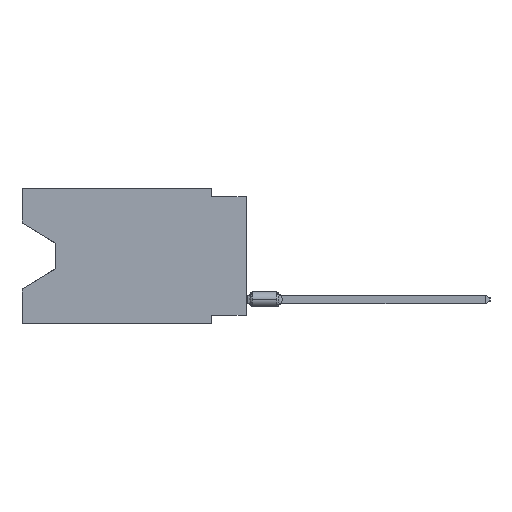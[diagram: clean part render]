
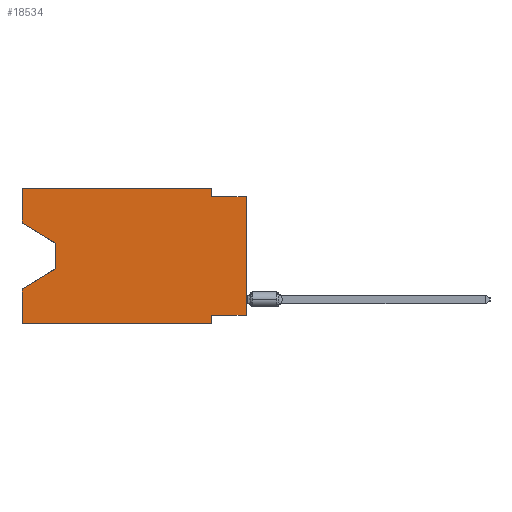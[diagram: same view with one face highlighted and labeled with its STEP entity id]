
A CAD part, left-side view. The second image highlights one B-rep face of the part: STEP entity #18534.
In plain terms, the highlighted planar face has unit normal (-1, 0, 0).
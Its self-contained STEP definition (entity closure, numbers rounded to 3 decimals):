
#212 = DIRECTION ( 'NONE',  ( 0., 0., -1. ) ) ;
#565 = EDGE_LOOP ( 'NONE', ( #54217, #32923, #70954, #8708, #57684, #69828, #55355, #9778, #17745, #63769, #45177, #51596 ) ) ;
#2578 = VECTOR ( 'NONE', #21114, 1000. ) ;
#3124 = VERTEX_POINT ( 'NONE', #63238 ) ;
#4812 = LINE ( 'NONE', #26596, #66347 ) ;
#5333 = VECTOR ( 'NONE', #43111, 1000. ) ;
#5863 = EDGE_CURVE ( 'NONE', #13954, #42335, #4812, .T. ) ;
#6368 = EDGE_CURVE ( 'NONE', #13954, #55034, #64513, .T. ) ;
#7191 = DIRECTION ( 'NONE',  ( 0., 0., 1. ) ) ;
#8708 = ORIENTED_EDGE ( 'NONE', *, *, #12662, .F. ) ;
#9778 = ORIENTED_EDGE ( 'NONE', *, *, #5863, .T. ) ;
#10524 = CARTESIAN_POINT ( 'NONE',  ( 0., 13.97, -5.893 ) ) ;
#10916 = VECTOR ( 'NONE', #31590, 1000. ) ;
#11325 = EDGE_CURVE ( 'NONE', #37197, #21861, #41984, .T. ) ;
#12066 = VECTOR ( 'NONE', #18634, 1000. ) ;
#12659 = CARTESIAN_POINT ( 'NONE',  ( 0., 16.383, -2.546 ) ) ;
#12662 = EDGE_CURVE ( 'NONE', #3124, #21861, #57821, .T. ) ;
#13291 = DIRECTION ( 'NONE',  ( 1., 0., 0. ) ) ;
#13871 = DIRECTION ( 'NONE',  ( 0., 1., 0. ) ) ;
#13954 = VERTEX_POINT ( 'NONE', #42633 ) ;
#14108 = VECTOR ( 'NONE', #62204, 1000. ) ;
#17097 = LINE ( 'NONE', #12659, #14108 ) ;
#17745 = ORIENTED_EDGE ( 'NONE', *, *, #31429, .F. ) ;
#18082 = LINE ( 'NONE', #69478, #70165 ) ;
#18534 = ADVANCED_FACE ( 'NONE', ( #29902 ), #41381, .F. ) ;
#18634 = DIRECTION ( 'NONE',  ( 0., -1., 0. ) ) ;
#18789 = LINE ( 'NONE', #30231, #33680 ) ;
#21114 = DIRECTION ( 'NONE',  ( 0., 0., 1. ) ) ;
#21443 = VERTEX_POINT ( 'NONE', #50872 ) ;
#21612 = LINE ( 'NONE', #39372, #64650 ) ;
#21861 = VERTEX_POINT ( 'NONE', #69190 ) ;
#22777 = EDGE_CURVE ( 'NONE', #52405, #71320, #17097, .T. ) ;
#23207 = LINE ( 'NONE', #46877, #46533 ) ;
#23223 = CARTESIAN_POINT ( 'NONE',  ( 0., 2.54, -9.906 ) ) ;
#23876 = EDGE_CURVE ( 'NONE', #71320, #37197, #21612, .T. ) ;
#26366 = CARTESIAN_POINT ( 'NONE',  ( 0., 0., -9.271 ) ) ;
#26596 = CARTESIAN_POINT ( 'NONE',  ( 0., 0., 0. ) ) ;
#29504 = DIRECTION ( 'NONE',  ( 0., 0., -1. ) ) ;
#29540 = DIRECTION ( 'NONE',  ( 0., 0., -1. ) ) ;
#29902 = FACE_OUTER_BOUND ( 'NONE', #565, .T. ) ;
#30231 = CARTESIAN_POINT ( 'NONE',  ( 0., 2.54, -9.906 ) ) ;
#31429 = EDGE_CURVE ( 'NONE', #60571, #42335, #18082, .T. ) ;
#31590 = DIRECTION ( 'NONE',  ( 0., 0.855, -0.519 ) ) ;
#31872 = EDGE_CURVE ( 'NONE', #21443, #60571, #47561, .T. ) ;
#32452 = CARTESIAN_POINT ( 'NONE',  ( 0., 16.383, 0. ) ) ;
#32923 = ORIENTED_EDGE ( 'NONE', *, *, #23876, .T. ) ;
#33680 = VECTOR ( 'NONE', #29504, 1000. ) ;
#37197 = VERTEX_POINT ( 'NONE', #65284 ) ;
#38465 = EDGE_CURVE ( 'NONE', #57218, #21443, #63375, .T. ) ;
#39372 = CARTESIAN_POINT ( 'NONE',  ( 0., 13.97, -4.013 ) ) ;
#40639 = DIRECTION ( 'NONE',  ( 0., -1., 0. ) ) ;
#41381 = PLANE ( 'NONE',  #57058 ) ;
#41984 = LINE ( 'NONE', #10524, #10916 ) ;
#42335 = VERTEX_POINT ( 'NONE', #71981 ) ;
#42633 = CARTESIAN_POINT ( 'NONE',  ( 0., 0., -9.271 ) ) ;
#43111 = DIRECTION ( 'NONE',  ( 0., 0., -1. ) ) ;
#45177 = ORIENTED_EDGE ( 'NONE', *, *, #38465, .F. ) ;
#45812 = CARTESIAN_POINT ( 'NONE',  ( 0., 2.54, -9.271 ) ) ;
#46135 = DIRECTION ( 'NONE',  ( 0., -1., 0. ) ) ;
#46533 = VECTOR ( 'NONE', #46135, 1000. ) ;
#46877 = CARTESIAN_POINT ( 'NONE',  ( 0., 16.383, -9.906 ) ) ;
#47561 = LINE ( 'NONE', #65660, #5333 ) ;
#50872 = CARTESIAN_POINT ( 'NONE',  ( 0., 2.54, 0. ) ) ;
#51596 = ORIENTED_EDGE ( 'NONE', *, *, #68145, .F. ) ;
#52257 = CARTESIAN_POINT ( 'NONE',  ( 0., 16.383, 0. ) ) ;
#52405 = VERTEX_POINT ( 'NONE', #56367 ) ;
#54217 = ORIENTED_EDGE ( 'NONE', *, *, #22777, .T. ) ;
#54415 = LINE ( 'NONE', #72112, #2578 ) ;
#55034 = VERTEX_POINT ( 'NONE', #45812 ) ;
#55355 = ORIENTED_EDGE ( 'NONE', *, *, #6368, .F. ) ;
#56367 = CARTESIAN_POINT ( 'NONE',  ( 0., 16.383, -2.546 ) ) ;
#57058 = AXIS2_PLACEMENT_3D ( 'NONE', #63934, #13291, #29540 ) ;
#57218 = VERTEX_POINT ( 'NONE', #32452 ) ;
#57684 = ORIENTED_EDGE ( 'NONE', *, *, #71118, .T. ) ;
#57821 = LINE ( 'NONE', #52257, #69174 ) ;
#57832 = CARTESIAN_POINT ( 'NONE',  ( 0., 16.383, 0. ) ) ;
#59981 = EDGE_CURVE ( 'NONE', #55034, #72298, #18789, .T. ) ;
#60545 = VECTOR ( 'NONE', #13871, 1000. ) ;
#60571 = VERTEX_POINT ( 'NONE', #61168 ) ;
#61168 = CARTESIAN_POINT ( 'NONE',  ( 0., 2.54, -0.635 ) ) ;
#61706 = DIRECTION ( 'NONE',  ( 0., 0., 1. ) ) ;
#62204 = DIRECTION ( 'NONE',  ( 0., -0.855, -0.519 ) ) ;
#63238 = CARTESIAN_POINT ( 'NONE',  ( 0., 16.383, -9.906 ) ) ;
#63375 = LINE ( 'NONE', #57832, #12066 ) ;
#63769 = ORIENTED_EDGE ( 'NONE', *, *, #31872, .F. ) ;
#63934 = CARTESIAN_POINT ( 'NONE',  ( 0., 16.383, 0. ) ) ;
#64513 = LINE ( 'NONE', #26366, #60545 ) ;
#64650 = VECTOR ( 'NONE', #212, 1000. ) ;
#65284 = CARTESIAN_POINT ( 'NONE',  ( 0., 13.97, -5.893 ) ) ;
#65660 = CARTESIAN_POINT ( 'NONE',  ( 0., 2.54, 0. ) ) ;
#66347 = VECTOR ( 'NONE', #61706, 1000. ) ;
#68145 = EDGE_CURVE ( 'NONE', #52405, #57218, #54415, .T. ) ;
#69174 = VECTOR ( 'NONE', #7191, 1000. ) ;
#69190 = CARTESIAN_POINT ( 'NONE',  ( 0., 16.383, -7.36 ) ) ;
#69478 = CARTESIAN_POINT ( 'NONE',  ( 0., 0., -0.635 ) ) ;
#69828 = ORIENTED_EDGE ( 'NONE', *, *, #59981, .F. ) ;
#70165 = VECTOR ( 'NONE', #40639, 1000. ) ;
#70839 = CARTESIAN_POINT ( 'NONE',  ( 0., 13.97, -4.013 ) ) ;
#70954 = ORIENTED_EDGE ( 'NONE', *, *, #11325, .T. ) ;
#71118 = EDGE_CURVE ( 'NONE', #3124, #72298, #23207, .T. ) ;
#71320 = VERTEX_POINT ( 'NONE', #70839 ) ;
#71981 = CARTESIAN_POINT ( 'NONE',  ( 0., 0., -0.635 ) ) ;
#72112 = CARTESIAN_POINT ( 'NONE',  ( 0., 16.383, 0. ) ) ;
#72298 = VERTEX_POINT ( 'NONE', #23223 ) ;
